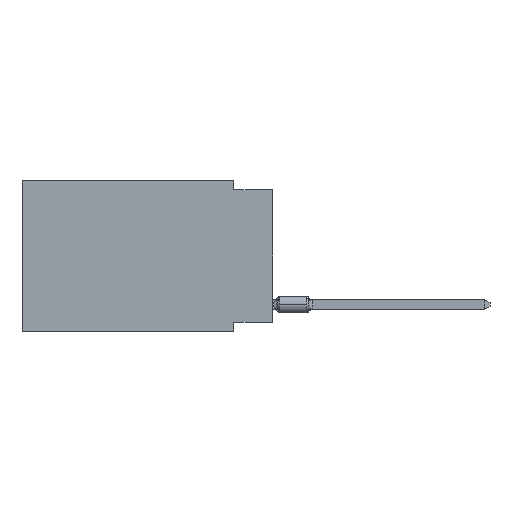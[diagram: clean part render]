
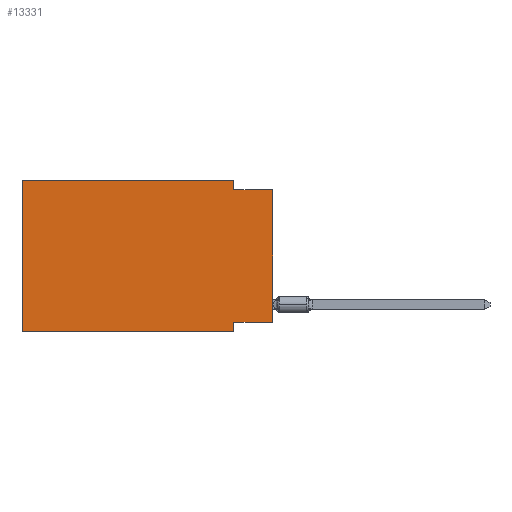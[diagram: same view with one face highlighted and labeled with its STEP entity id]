
A CAD part, left-side view. The second image highlights one B-rep face of the part: STEP entity #13331.
In plain terms, the highlighted planar face has unit normal (-1, 0, 0).
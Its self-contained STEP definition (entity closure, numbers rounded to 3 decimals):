
#126 = CARTESIAN_POINT ( 'NONE',  ( 0., 0., 0. ) ) ;
#278 = DIRECTION ( 'NONE',  ( 0., 0., -1. ) ) ;
#442 = VERTEX_POINT ( 'NONE', #22422 ) ;
#658 = EDGE_CURVE ( 'NONE', #442, #12801, #1512, .T. ) ;
#991 = ORIENTED_EDGE ( 'NONE', *, *, #21194, .T. ) ;
#1243 = CARTESIAN_POINT ( 'NONE',  ( 0., 2.54, 0. ) ) ;
#1512 = LINE ( 'NONE', #18051, #10985 ) ;
#1733 = EDGE_CURVE ( 'NONE', #12801, #1888, #7071, .T. ) ;
#1843 = EDGE_CURVE ( 'NONE', #1949, #15812, #11522, .T. ) ;
#1846 = DIRECTION ( 'NONE',  ( 0., 1., 0. ) ) ;
#1888 = VERTEX_POINT ( 'NONE', #20999 ) ;
#1949 = VERTEX_POINT ( 'NONE', #4550 ) ;
#2394 = DIRECTION ( 'NONE',  ( 0., 0., 1. ) ) ;
#3599 = LINE ( 'NONE', #16768, #16701 ) ;
#4550 = CARTESIAN_POINT ( 'NONE',  ( 0., 0., -9.271 ) ) ;
#4748 = EDGE_LOOP ( 'NONE', ( #17980, #21956, #10819, #16742, #6538, #991, #10515, #18019 ) ) ;
#4879 = FACE_OUTER_BOUND ( 'NONE', #4748, .T. ) ;
#4919 = VECTOR ( 'NONE', #5827, 1000. ) ;
#4975 = DIRECTION ( 'NONE',  ( 0., 0., 1. ) ) ;
#5111 = PLANE ( 'NONE',  #20517 ) ;
#5568 = VECTOR ( 'NONE', #278, 1000. ) ;
#5827 = DIRECTION ( 'NONE',  ( 0., -1., 0. ) ) ;
#6253 = EDGE_CURVE ( 'NONE', #1949, #19767, #6979, .T. ) ;
#6538 = ORIENTED_EDGE ( 'NONE', *, *, #658, .F. ) ;
#6676 = CARTESIAN_POINT ( 'NONE',  ( 0., 16.383, 0. ) ) ;
#6895 = CARTESIAN_POINT ( 'NONE',  ( 0., 2.54, -0.635 ) ) ;
#6979 = LINE ( 'NONE', #7227, #8199 ) ;
#7071 = LINE ( 'NONE', #10803, #19271 ) ;
#7227 = CARTESIAN_POINT ( 'NONE',  ( 0., 0., -9.271 ) ) ;
#7255 = CARTESIAN_POINT ( 'NONE',  ( 0., 0., -0.635 ) ) ;
#8105 = EDGE_CURVE ( 'NONE', #1888, #18801, #19605, .T. ) ;
#8199 = VECTOR ( 'NONE', #1846, 1000. ) ;
#8437 = VERTEX_POINT ( 'NONE', #21037 ) ;
#9042 = DIRECTION ( 'NONE',  ( 0., 0., -1. ) ) ;
#9626 = CARTESIAN_POINT ( 'NONE',  ( 0., 2.54, -9.906 ) ) ;
#10101 = VECTOR ( 'NONE', #2394, 1000. ) ;
#10515 = ORIENTED_EDGE ( 'NONE', *, *, #20925, .F. ) ;
#10803 = CARTESIAN_POINT ( 'NONE',  ( 0., 16.383, 0. ) ) ;
#10819 = ORIENTED_EDGE ( 'NONE', *, *, #8105, .F. ) ;
#10985 = VECTOR ( 'NONE', #4975, 1000. ) ;
#11133 = LINE ( 'NONE', #15077, #4919 ) ;
#11522 = LINE ( 'NONE', #126, #10101 ) ;
#12556 = DIRECTION ( 'NONE',  ( 0., 0., -1. ) ) ;
#12801 = VERTEX_POINT ( 'NONE', #15251 ) ;
#13331 = ADVANCED_FACE ( 'NONE', ( #4879 ), #5111, .F. ) ;
#14405 = DIRECTION ( 'NONE',  ( 0., -1., 0. ) ) ;
#15077 = CARTESIAN_POINT ( 'NONE',  ( 0., 0., -0.635 ) ) ;
#15251 = CARTESIAN_POINT ( 'NONE',  ( 0., 16.383, 0. ) ) ;
#15812 = VERTEX_POINT ( 'NONE', #7255 ) ;
#16701 = VECTOR ( 'NONE', #23535, 1000. ) ;
#16716 = LINE ( 'NONE', #9626, #5568 ) ;
#16742 = ORIENTED_EDGE ( 'NONE', *, *, #1733, .F. ) ;
#16768 = CARTESIAN_POINT ( 'NONE',  ( 0., 16.383, -9.906 ) ) ;
#17790 = VECTOR ( 'NONE', #9042, 1000. ) ;
#17980 = ORIENTED_EDGE ( 'NONE', *, *, #1843, .T. ) ;
#18019 = ORIENTED_EDGE ( 'NONE', *, *, #6253, .F. ) ;
#18051 = CARTESIAN_POINT ( 'NONE',  ( 0., 16.383, 0. ) ) ;
#18801 = VERTEX_POINT ( 'NONE', #6895 ) ;
#19271 = VECTOR ( 'NONE', #14405, 1000. ) ;
#19531 = DIRECTION ( 'NONE',  ( 1., 0., 0. ) ) ;
#19605 = LINE ( 'NONE', #1243, #17790 ) ;
#19767 = VERTEX_POINT ( 'NONE', #19879 ) ;
#19879 = CARTESIAN_POINT ( 'NONE',  ( 0., 2.54, -9.271 ) ) ;
#20517 = AXIS2_PLACEMENT_3D ( 'NONE', #6676, #19531, #12556 ) ;
#20925 = EDGE_CURVE ( 'NONE', #19767, #8437, #16716, .T. ) ;
#20999 = CARTESIAN_POINT ( 'NONE',  ( 0., 2.54, 0. ) ) ;
#21037 = CARTESIAN_POINT ( 'NONE',  ( 0., 2.54, -9.906 ) ) ;
#21194 = EDGE_CURVE ( 'NONE', #442, #8437, #3599, .T. ) ;
#21956 = ORIENTED_EDGE ( 'NONE', *, *, #23006, .F. ) ;
#22422 = CARTESIAN_POINT ( 'NONE',  ( 0., 16.383, -9.906 ) ) ;
#23006 = EDGE_CURVE ( 'NONE', #18801, #15812, #11133, .T. ) ;
#23535 = DIRECTION ( 'NONE',  ( 0., -1., 0. ) ) ;
